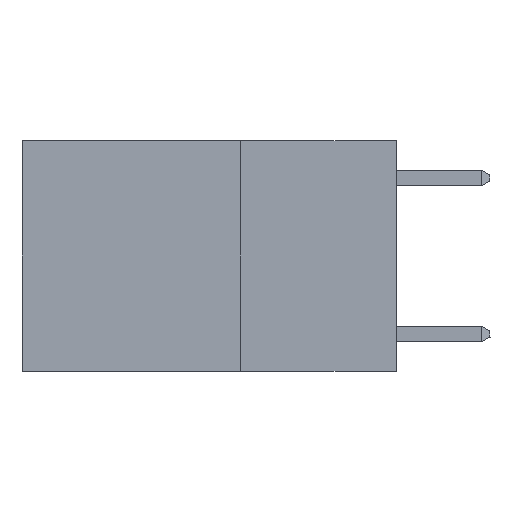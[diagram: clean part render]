
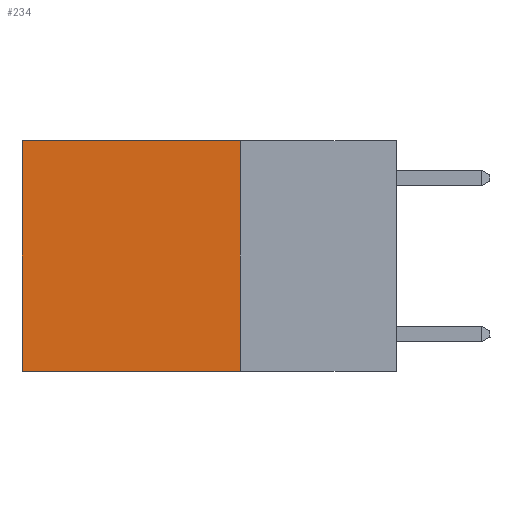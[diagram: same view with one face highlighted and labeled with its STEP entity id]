
A CAD part, left-side view. The second image highlights one B-rep face of the part: STEP entity #234.
In plain terms, the highlighted planar face has unit normal (-1, 0, 0).
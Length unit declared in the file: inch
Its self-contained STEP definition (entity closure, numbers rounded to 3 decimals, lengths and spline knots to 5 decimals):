
#104 = VERTEX_POINT ( 'NONE', #8831 ) ;
#234 = ADVANCED_FACE ( 'NONE', ( #13787 ), #3268, .F. ) ;
#576 = CARTESIAN_POINT ( 'NONE',  ( 0.2625, 0.25, 0. ) ) ;
#1116 = EDGE_CURVE ( 'NONE', #9684, #9156, #14988, .T. ) ;
#1368 = CARTESIAN_POINT ( 'NONE',  ( 0.2625, 0.6, -0.37 ) ) ;
#1897 = VECTOR ( 'NONE', #9803, 39.37008 ) ;
#3268 = PLANE ( 'NONE',  #14784 ) ;
#3434 = DIRECTION ( 'NONE',  ( 0., 0., -1. ) ) ;
#4050 = CARTESIAN_POINT ( 'NONE',  ( 0.2625, 0.6, 0. ) ) ;
#4151 = EDGE_CURVE ( 'NONE', #4222, #104, #11021, .T. ) ;
#4189 = EDGE_CURVE ( 'NONE', #104, #9156, #14335, .T. ) ;
#4222 = VERTEX_POINT ( 'NONE', #576 ) ;
#4387 = DIRECTION ( 'NONE',  ( 0., 1., 0. ) ) ;
#4439 = CARTESIAN_POINT ( 'NONE',  ( 0.2625, 0.25, 0. ) ) ;
#5137 = DIRECTION ( 'NONE',  ( 0., 1., 0. ) ) ;
#5753 = DIRECTION ( 'NONE',  ( 1., 0., 0. ) ) ;
#6588 = VECTOR ( 'NONE', #5137, 39.37008 ) ;
#6674 = DIRECTION ( 'NONE',  ( 0., 0., -1. ) ) ;
#6850 = CARTESIAN_POINT ( 'NONE',  ( 0.2625, 0.25, -0.37 ) ) ;
#6932 = ORIENTED_EDGE ( 'NONE', *, *, #1116, .F. ) ;
#7462 = VECTOR ( 'NONE', #4387, 39.37008 ) ;
#8346 = ORIENTED_EDGE ( 'NONE', *, *, #4151, .T. ) ;
#8679 = ORIENTED_EDGE ( 'NONE', *, *, #4189, .T. ) ;
#8831 = CARTESIAN_POINT ( 'NONE',  ( 0.2625, 0.6, 0. ) ) ;
#9041 = VECTOR ( 'NONE', #3434, 39.37008 ) ;
#9156 = VERTEX_POINT ( 'NONE', #1368 ) ;
#9553 = ORIENTED_EDGE ( 'NONE', *, *, #14931, .F. ) ;
#9684 = VERTEX_POINT ( 'NONE', #12857 ) ;
#9803 = DIRECTION ( 'NONE',  ( 0., 0., -1. ) ) ;
#11021 = LINE ( 'NONE', #13462, #6588 ) ;
#11498 = CARTESIAN_POINT ( 'NONE',  ( 0.2625, 0.25, 0. ) ) ;
#12857 = CARTESIAN_POINT ( 'NONE',  ( 0.2625, 0.25, -0.37 ) ) ;
#13462 = CARTESIAN_POINT ( 'NONE',  ( 0.2625, 0.25, 0. ) ) ;
#13787 = FACE_OUTER_BOUND ( 'NONE', #13874, .T. ) ;
#13874 = EDGE_LOOP ( 'NONE', ( #8679, #6932, #9553, #8346 ) ) ;
#13943 = LINE ( 'NONE', #4439, #9041 ) ;
#14335 = LINE ( 'NONE', #4050, #1897 ) ;
#14784 = AXIS2_PLACEMENT_3D ( 'NONE', #11498, #5753, #6674 ) ;
#14931 = EDGE_CURVE ( 'NONE', #4222, #9684, #13943, .T. ) ;
#14988 = LINE ( 'NONE', #6850, #7462 ) ;
